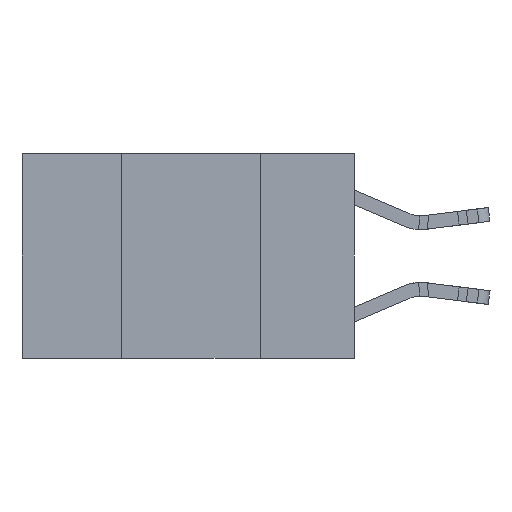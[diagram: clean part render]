
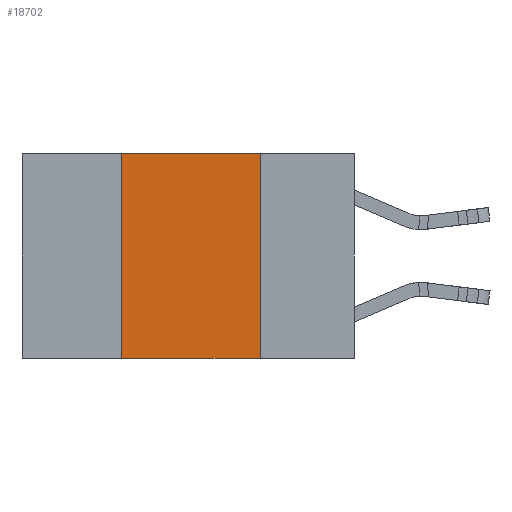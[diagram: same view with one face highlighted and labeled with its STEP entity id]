
A CAD part, left-side view. The second image highlights one B-rep face of the part: STEP entity #18702.
In plain terms, the highlighted planar face has unit normal (-1, 0, 0).
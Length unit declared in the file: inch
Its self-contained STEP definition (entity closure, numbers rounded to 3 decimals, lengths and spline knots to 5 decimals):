
#50 = ORIENTED_EDGE ( 'NONE', *, *, #10712, .T. ) ;
#317 = FACE_OUTER_BOUND ( 'NONE', #15513, .T. ) ;
#1717 = PLANE ( 'NONE',  #18269 ) ;
#3956 = VERTEX_POINT ( 'NONE', #28753 ) ;
#4193 = CARTESIAN_POINT ( 'NONE',  ( 0., 0.6, -0.37 ) ) ;
#4405 = DIRECTION ( 'NONE',  ( 0., 0., 1. ) ) ;
#5287 = CARTESIAN_POINT ( 'NONE',  ( 0., 0.42, -0.37 ) ) ;
#5960 = LINE ( 'NONE', #11460, #12935 ) ;
#6246 = CARTESIAN_POINT ( 'NONE',  ( 0., 0.6, 0. ) ) ;
#6478 = DIRECTION ( 'NONE',  ( 1., 0., 0. ) ) ;
#9778 = VECTOR ( 'NONE', #27496, 39.37008 ) ;
#10712 = EDGE_CURVE ( 'NONE', #12488, #3956, #16661, .T. ) ;
#11460 = CARTESIAN_POINT ( 'NONE',  ( 0., 0.17, 0. ) ) ;
#11846 = ORIENTED_EDGE ( 'NONE', *, *, #22161, .F. ) ;
#12189 = VECTOR ( 'NONE', #22520, 39.37008 ) ;
#12269 = EDGE_CURVE ( 'NONE', #13410, #3956, #5960, .T. ) ;
#12488 = VERTEX_POINT ( 'NONE', #5287 ) ;
#12935 = VECTOR ( 'NONE', #25452, 39.37008 ) ;
#13410 = VERTEX_POINT ( 'NONE', #26889 ) ;
#13506 = EDGE_CURVE ( 'NONE', #22606, #13410, #22321, .T. ) ;
#15513 = EDGE_LOOP ( 'NONE', ( #21972, #16554, #11846, #50 ) ) ;
#16554 = ORIENTED_EDGE ( 'NONE', *, *, #13506, .F. ) ;
#16661 = LINE ( 'NONE', #4193, #9778 ) ;
#17458 = CARTESIAN_POINT ( 'NONE',  ( 0., 0.42, 0. ) ) ;
#18269 = AXIS2_PLACEMENT_3D ( 'NONE', #20417, #6478, #22734 ) ;
#18702 = ADVANCED_FACE ( 'NONE', ( #317 ), #1717, .F. ) ;
#20417 = CARTESIAN_POINT ( 'NONE',  ( 0., 0.6, 0. ) ) ;
#21972 = ORIENTED_EDGE ( 'NONE', *, *, #12269, .F. ) ;
#22161 = EDGE_CURVE ( 'NONE', #12488, #22606, #23859, .T. ) ;
#22321 = LINE ( 'NONE', #6246, #12189 ) ;
#22520 = DIRECTION ( 'NONE',  ( 0., -1., 0. ) ) ;
#22606 = VERTEX_POINT ( 'NONE', #17458 ) ;
#22734 = DIRECTION ( 'NONE',  ( 0., 0., -1. ) ) ;
#23105 = VECTOR ( 'NONE', #4405, 39.37008 ) ;
#23859 = LINE ( 'NONE', #25391, #23105 ) ;
#25391 = CARTESIAN_POINT ( 'NONE',  ( 0., 0.42, 0. ) ) ;
#25452 = DIRECTION ( 'NONE',  ( 0., 0., -1. ) ) ;
#26889 = CARTESIAN_POINT ( 'NONE',  ( 0., 0.17, 0. ) ) ;
#27496 = DIRECTION ( 'NONE',  ( 0., -1., 0. ) ) ;
#28753 = CARTESIAN_POINT ( 'NONE',  ( 0., 0.17, -0.37 ) ) ;
